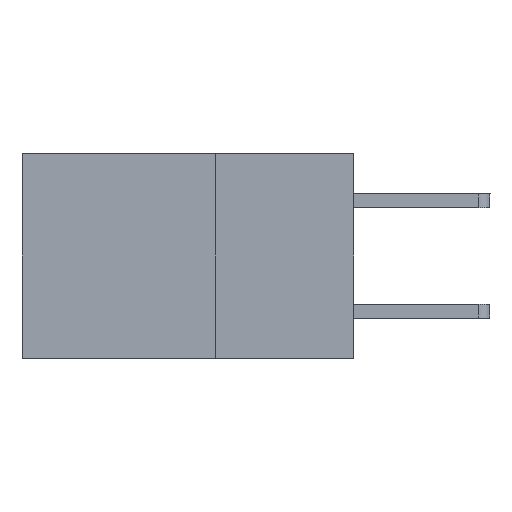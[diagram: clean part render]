
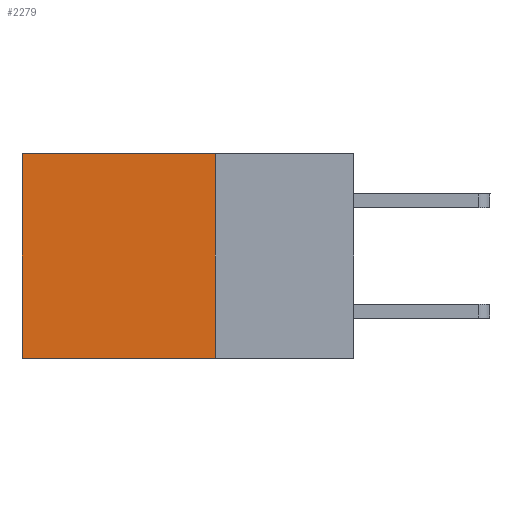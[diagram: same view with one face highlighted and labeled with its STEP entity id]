
A CAD part, left-side view. The second image highlights one B-rep face of the part: STEP entity #2279.
In plain terms, the highlighted planar face has unit normal (-1, 0, 0).
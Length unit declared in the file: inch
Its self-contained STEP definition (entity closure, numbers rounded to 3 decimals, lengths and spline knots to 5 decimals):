
#167 = ORIENTED_EDGE ( 'NONE', *, *, #6352, .T. ) ;
#379 = LINE ( 'NONE', #9858, #13961 ) ;
#595 = VERTEX_POINT ( 'NONE', #7043 ) ;
#872 = LINE ( 'NONE', #2072, #6955 ) ;
#916 = VERTEX_POINT ( 'NONE', #9911 ) ;
#994 = CARTESIAN_POINT ( 'NONE',  ( 0.2875, 0.25, 0. ) ) ;
#1122 = EDGE_CURVE ( 'NONE', #8481, #595, #872, .T. ) ;
#1389 = CARTESIAN_POINT ( 'NONE',  ( 0.2875, 0.25, 0. ) ) ;
#2072 = CARTESIAN_POINT ( 'NONE',  ( 0.2875, 0.25, 0. ) ) ;
#2205 = CARTESIAN_POINT ( 'NONE',  ( 0.2875, 0.25, 0. ) ) ;
#2279 = ADVANCED_FACE ( 'NONE', ( #4057 ), #8598, .F. ) ;
#3490 = DIRECTION ( 'NONE',  ( 1., 0., 0. ) ) ;
#3593 = VECTOR ( 'NONE', #5732, 39.37008 ) ;
#3728 = ORIENTED_EDGE ( 'NONE', *, *, #1122, .T. ) ;
#3784 = DIRECTION ( 'NONE',  ( 0., 1., 0. ) ) ;
#3790 = VECTOR ( 'NONE', #3784, 39.37008 ) ;
#4057 = FACE_OUTER_BOUND ( 'NONE', #8382, .T. ) ;
#4951 = LINE ( 'NONE', #9191, #3790 ) ;
#5244 = CARTESIAN_POINT ( 'NONE',  ( 0.2875, 0.25, -0.37 ) ) ;
#5732 = DIRECTION ( 'NONE',  ( 0., 0., -1. ) ) ;
#6352 = EDGE_CURVE ( 'NONE', #595, #916, #379, .T. ) ;
#6839 = EDGE_CURVE ( 'NONE', #8481, #10434, #9832, .T. ) ;
#6955 = VECTOR ( 'NONE', #7498, 39.37008 ) ;
#7043 = CARTESIAN_POINT ( 'NONE',  ( 0.2875, 0.6, 0. ) ) ;
#7498 = DIRECTION ( 'NONE',  ( 0., 1., 0. ) ) ;
#7547 = DIRECTION ( 'NONE',  ( 0., 0., -1. ) ) ;
#8253 = EDGE_CURVE ( 'NONE', #10434, #916, #4951, .T. ) ;
#8382 = EDGE_LOOP ( 'NONE', ( #167, #13953, #9329, #3728 ) ) ;
#8481 = VERTEX_POINT ( 'NONE', #2205 ) ;
#8598 = PLANE ( 'NONE',  #10948 ) ;
#9191 = CARTESIAN_POINT ( 'NONE',  ( 0.2875, 0.25, -0.37 ) ) ;
#9329 = ORIENTED_EDGE ( 'NONE', *, *, #6839, .F. ) ;
#9832 = LINE ( 'NONE', #1389, #3593 ) ;
#9858 = CARTESIAN_POINT ( 'NONE',  ( 0.2875, 0.6, 0. ) ) ;
#9911 = CARTESIAN_POINT ( 'NONE',  ( 0.2875, 0.6, -0.37 ) ) ;
#10434 = VERTEX_POINT ( 'NONE', #5244 ) ;
#10948 = AXIS2_PLACEMENT_3D ( 'NONE', #994, #3490, #7547 ) ;
#13400 = DIRECTION ( 'NONE',  ( 0., 0., -1. ) ) ;
#13953 = ORIENTED_EDGE ( 'NONE', *, *, #8253, .F. ) ;
#13961 = VECTOR ( 'NONE', #13400, 39.37008 ) ;
